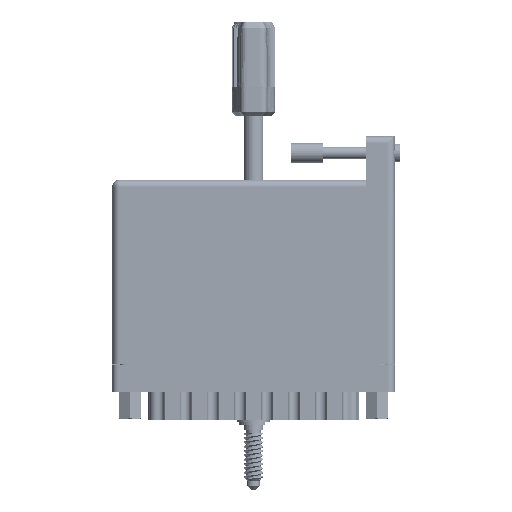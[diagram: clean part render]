
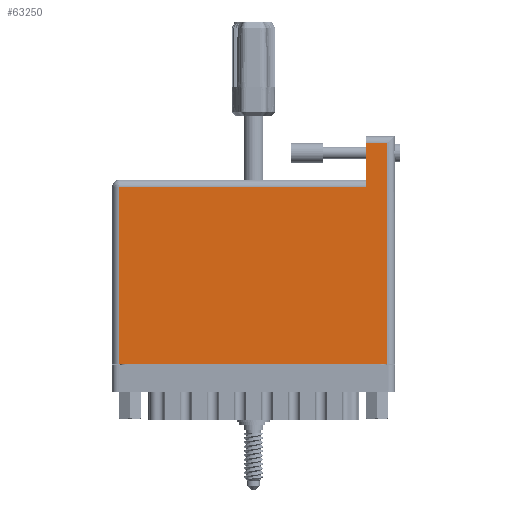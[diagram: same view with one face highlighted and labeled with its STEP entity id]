
A CAD part, front view. The second image highlights one B-rep face of the part: STEP entity #63250.
In plain terms, the highlighted face is planar.
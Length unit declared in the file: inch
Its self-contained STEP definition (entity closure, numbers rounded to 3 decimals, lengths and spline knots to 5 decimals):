
#408 = ORIENTED_EDGE ( 'NONE', *, *, #83607, .T. ) ;
#1271 = LINE ( 'NONE', #7276, #27478 ) ;
#2087 = VERTEX_POINT ( 'NONE', #84511 ) ;
#4814 = ORIENTED_EDGE ( 'NONE', *, *, #51352, .T. ) ;
#4985 = EDGE_CURVE ( 'NONE', #85375, #42163, #67662, .T. ) ;
#5748 = ORIENTED_EDGE ( 'NONE', *, *, #9640, .T. ) ;
#7276 = CARTESIAN_POINT ( 'NONE',  ( 0., 2.125, 0. ) ) ;
#8260 = CARTESIAN_POINT ( 'NONE',  ( 0.07, 1.705, 0. ) ) ;
#9640 = EDGE_CURVE ( 'NONE', #32209, #78370, #57885, .T. ) ;
#11160 = ORIENTED_EDGE ( 'NONE', *, *, #98825, .T. ) ;
#15553 = VECTOR ( 'NONE', #49586, 39.37008 ) ;
#18441 = DIRECTION ( 'NONE',  ( -1., 0., 0. ) ) ;
#24570 = VERTEX_POINT ( 'NONE', #92295 ) ;
#25105 = CARTESIAN_POINT ( 'NONE',  ( 0.07, 0., 0. ) ) ;
#25306 = CARTESIAN_POINT ( 'NONE',  ( 2.438, 2.125, 0. ) ) ;
#27478 = VECTOR ( 'NONE', #31746, 39.37008 ) ;
#27877 = AXIS2_PLACEMENT_3D ( 'NONE', #32973, #62525, #63023 ) ;
#28374 = ORIENTED_EDGE ( 'NONE', *, *, #33669, .T. ) ;
#31746 = DIRECTION ( 'NONE',  ( -1., 0., 0. ) ) ;
#32209 = VERTEX_POINT ( 'NONE', #25306 ) ;
#32904 = CARTESIAN_POINT ( 'NONE',  ( 2.438, 2.195, 0. ) ) ;
#32973 = CARTESIAN_POINT ( 'NONE',  ( 0., 1.775, 0. ) ) ;
#33669 = EDGE_CURVE ( 'NONE', #2087, #24570, #63493, .T. ) ;
#39361 = CARTESIAN_POINT ( 'NONE',  ( 2.438, 1.705, 0. ) ) ;
#42163 = VERTEX_POINT ( 'NONE', #91219 ) ;
#48119 = CARTESIAN_POINT ( 'NONE',  ( 0., 0., 0. ) ) ;
#49554 = EDGE_LOOP ( 'NONE', ( #11160, #93725, #408, #28374, #4814, #5748 ) ) ;
#49586 = DIRECTION ( 'NONE',  ( 1., 0., 0. ) ) ;
#49934 = CARTESIAN_POINT ( 'NONE',  ( 0., 1.705, 0. ) ) ;
#51352 = EDGE_CURVE ( 'NONE', #24570, #32209, #1271, .T. ) ;
#55638 = LINE ( 'NONE', #48119, #15553 ) ;
#56964 = CARTESIAN_POINT ( 'NONE',  ( 2.648, 2.195, 0. ) ) ;
#57885 = LINE ( 'NONE', #32904, #92240 ) ;
#62525 = DIRECTION ( 'NONE',  ( 0., 0., -1. ) ) ;
#63023 = DIRECTION ( 'NONE',  ( -1., 0., 0. ) ) ;
#63250 = ADVANCED_FACE ( 'NONE', ( #70508 ), #87494, .F. ) ;
#63493 = LINE ( 'NONE', #56964, #66281 ) ;
#66281 = VECTOR ( 'NONE', #86982, 39.37008 ) ;
#67662 = LINE ( 'NONE', #25105, #96017 ) ;
#68996 = VECTOR ( 'NONE', #18441, 39.37008 ) ;
#70508 = FACE_OUTER_BOUND ( 'NONE', #49554, .T. ) ;
#71124 = DIRECTION ( 'NONE',  ( 0., -1., 0. ) ) ;
#78370 = VERTEX_POINT ( 'NONE', #39361 ) ;
#79409 = DIRECTION ( 'NONE',  ( 0., -1., 0. ) ) ;
#83607 = EDGE_CURVE ( 'NONE', #42163, #2087, #55638, .T. ) ;
#84511 = CARTESIAN_POINT ( 'NONE',  ( 2.648, 0., 0. ) ) ;
#85375 = VERTEX_POINT ( 'NONE', #8260 ) ;
#86982 = DIRECTION ( 'NONE',  ( 0., 1., 0. ) ) ;
#87494 = PLANE ( 'NONE',  #27877 ) ;
#91219 = CARTESIAN_POINT ( 'NONE',  ( 0.07, 0., 0. ) ) ;
#92240 = VECTOR ( 'NONE', #79409, 39.37008 ) ;
#92295 = CARTESIAN_POINT ( 'NONE',  ( 2.648, 2.125, 0. ) ) ;
#93725 = ORIENTED_EDGE ( 'NONE', *, *, #4985, .T. ) ;
#94973 = LINE ( 'NONE', #49934, #68996 ) ;
#96017 = VECTOR ( 'NONE', #71124, 39.37008 ) ;
#98825 = EDGE_CURVE ( 'NONE', #78370, #85375, #94973, .T. ) ;
